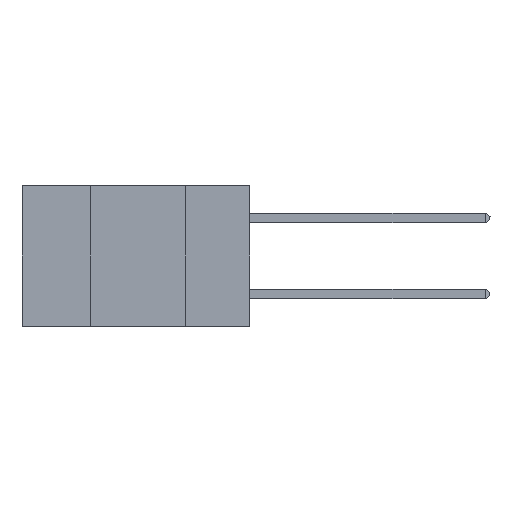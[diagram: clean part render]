
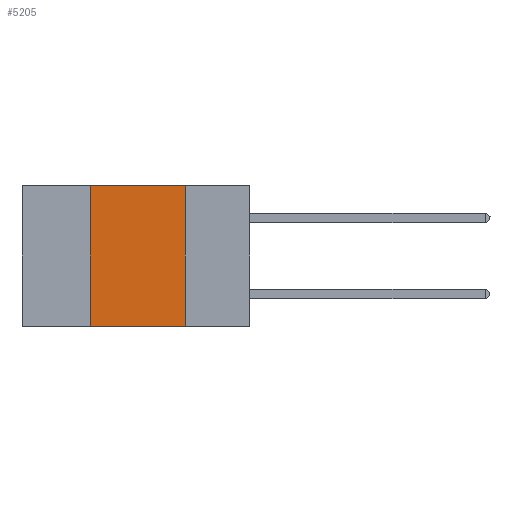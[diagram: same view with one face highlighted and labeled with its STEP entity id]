
A CAD part, left-side view. The second image highlights one B-rep face of the part: STEP entity #5205.
In plain terms, the highlighted planar face has unit normal (-1, 0, 0).
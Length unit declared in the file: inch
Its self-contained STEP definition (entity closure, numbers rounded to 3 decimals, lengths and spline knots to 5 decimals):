
#764 = EDGE_CURVE ( 'NONE', #9854, #22341, #23842, .T. ) ;
#949 = VECTOR ( 'NONE', #10620, 39.37008 ) ;
#1723 = ORIENTED_EDGE ( 'NONE', *, *, #11572, .T. ) ;
#2436 = DIRECTION ( 'NONE',  ( 1., 0., 0. ) ) ;
#4174 = EDGE_CURVE ( 'NONE', #22341, #16440, #21108, .T. ) ;
#5205 = ADVANCED_FACE ( 'NONE', ( #17137 ), #10883, .F. ) ;
#5387 = VECTOR ( 'NONE', #19495, 39.37008 ) ;
#6776 = CARTESIAN_POINT ( 'NONE',  ( 0., 0.42, -0.37 ) ) ;
#7357 = ORIENTED_EDGE ( 'NONE', *, *, #764, .F. ) ;
#7538 = ORIENTED_EDGE ( 'NONE', *, *, #4174, .F. ) ;
#7580 = DIRECTION ( 'NONE',  ( 0., 0., -1. ) ) ;
#8311 = LINE ( 'NONE', #16564, #16097 ) ;
#9854 = VERTEX_POINT ( 'NONE', #6776 ) ;
#9969 = LINE ( 'NONE', #22585, #16472 ) ;
#10157 = DIRECTION ( 'NONE',  ( 0., -1., 0. ) ) ;
#10353 = EDGE_CURVE ( 'NONE', #16440, #12543, #9969, .T. ) ;
#10620 = DIRECTION ( 'NONE',  ( 0., -1., 0. ) ) ;
#10883 = PLANE ( 'NONE',  #25691 ) ;
#11018 = DIRECTION ( 'NONE',  ( 0., 0., -1. ) ) ;
#11572 = EDGE_CURVE ( 'NONE', #9854, #12543, #8311, .T. ) ;
#12283 = CARTESIAN_POINT ( 'NONE',  ( 0., 0.6, 0. ) ) ;
#12293 = EDGE_LOOP ( 'NONE', ( #22076, #7538, #7357, #1723 ) ) ;
#12543 = VERTEX_POINT ( 'NONE', #27447 ) ;
#16097 = VECTOR ( 'NONE', #10157, 39.37008 ) ;
#16440 = VERTEX_POINT ( 'NONE', #21585 ) ;
#16472 = VECTOR ( 'NONE', #7580, 39.37008 ) ;
#16564 = CARTESIAN_POINT ( 'NONE',  ( 0., 0.6, -0.37 ) ) ;
#17137 = FACE_OUTER_BOUND ( 'NONE', #12293, .T. ) ;
#17886 = CARTESIAN_POINT ( 'NONE',  ( 0., 0.42, 0. ) ) ;
#19495 = DIRECTION ( 'NONE',  ( 0., 0., 1. ) ) ;
#21108 = LINE ( 'NONE', #12283, #949 ) ;
#21585 = CARTESIAN_POINT ( 'NONE',  ( 0., 0.17, 0. ) ) ;
#21653 = CARTESIAN_POINT ( 'NONE',  ( 0., 0.6, 0. ) ) ;
#22076 = ORIENTED_EDGE ( 'NONE', *, *, #10353, .F. ) ;
#22341 = VERTEX_POINT ( 'NONE', #24581 ) ;
#22585 = CARTESIAN_POINT ( 'NONE',  ( 0., 0.17, 0. ) ) ;
#23842 = LINE ( 'NONE', #17886, #5387 ) ;
#24581 = CARTESIAN_POINT ( 'NONE',  ( 0., 0.42, 0. ) ) ;
#25691 = AXIS2_PLACEMENT_3D ( 'NONE', #21653, #2436, #11018 ) ;
#27447 = CARTESIAN_POINT ( 'NONE',  ( 0., 0.17, -0.37 ) ) ;
